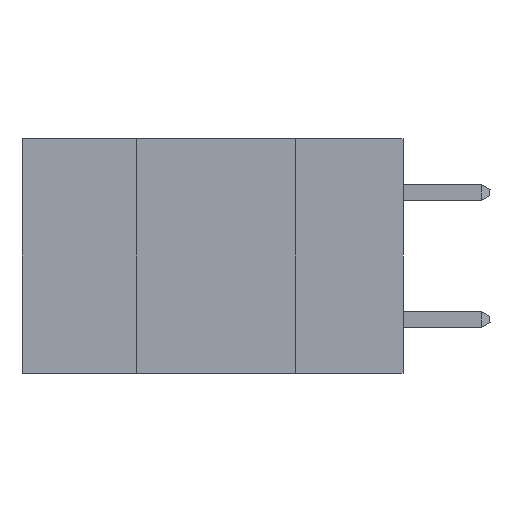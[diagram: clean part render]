
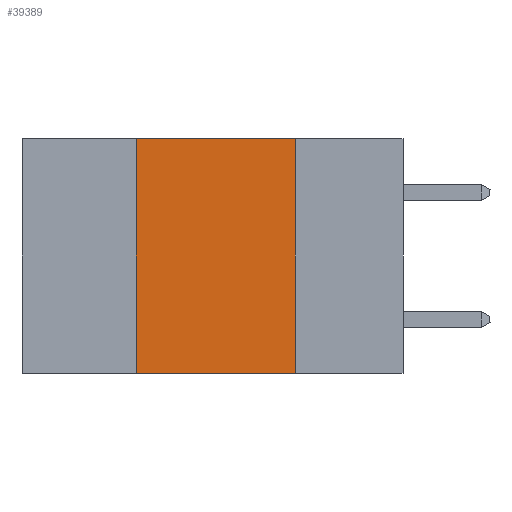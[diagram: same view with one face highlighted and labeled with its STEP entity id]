
A CAD part, left-side view. The second image highlights one B-rep face of the part: STEP entity #39389.
In plain terms, the highlighted planar face has unit normal (-1, 0, 0).
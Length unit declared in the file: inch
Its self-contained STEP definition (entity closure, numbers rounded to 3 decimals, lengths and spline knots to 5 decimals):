
#234 = CARTESIAN_POINT ( 'NONE',  ( 0., 0.6, 0. ) ) ;
#533 = PLANE ( 'NONE',  #46203 ) ;
#936 = ORIENTED_EDGE ( 'NONE', *, *, #8516, .T. ) ;
#1502 = ORIENTED_EDGE ( 'NONE', *, *, #2076, .F. ) ;
#1840 = EDGE_LOOP ( 'NONE', ( #38169, #26956, #1502, #936 ) ) ;
#2076 = EDGE_CURVE ( 'NONE', #39850, #3855, #32888, .T. ) ;
#2745 = DIRECTION ( 'NONE',  ( 0., 0., -1. ) ) ;
#3281 = CARTESIAN_POINT ( 'NONE',  ( 0., 0.17, -0.37 ) ) ;
#3855 = VERTEX_POINT ( 'NONE', #32870 ) ;
#5832 = DIRECTION ( 'NONE',  ( 0., -1., 0. ) ) ;
#7295 = DIRECTION ( 'NONE',  ( 0., -1., 0. ) ) ;
#8516 = EDGE_CURVE ( 'NONE', #39850, #12502, #23339, .T. ) ;
#12502 = VERTEX_POINT ( 'NONE', #3281 ) ;
#12785 = CARTESIAN_POINT ( 'NONE',  ( 0., 0.6, -0.37 ) ) ;
#13663 = VECTOR ( 'NONE', #21708, 39.37008 ) ;
#14873 = VECTOR ( 'NONE', #5832, 39.37008 ) ;
#16962 = CARTESIAN_POINT ( 'NONE',  ( 0., 0.42, -0.37 ) ) ;
#18075 = CARTESIAN_POINT ( 'NONE',  ( 0., 0.42, 0. ) ) ;
#19120 = EDGE_CURVE ( 'NONE', #3855, #32318, #36727, .T. ) ;
#21708 = DIRECTION ( 'NONE',  ( 0., 0., 1. ) ) ;
#23339 = LINE ( 'NONE', #12785, #14873 ) ;
#25687 = DIRECTION ( 'NONE',  ( 0., 0., -1. ) ) ;
#26317 = CARTESIAN_POINT ( 'NONE',  ( 0., 0.17, 0. ) ) ;
#26956 = ORIENTED_EDGE ( 'NONE', *, *, #19120, .F. ) ;
#31053 = VECTOR ( 'NONE', #7295, 39.37008 ) ;
#32318 = VERTEX_POINT ( 'NONE', #26317 ) ;
#32870 = CARTESIAN_POINT ( 'NONE',  ( 0., 0.42, 0. ) ) ;
#32888 = LINE ( 'NONE', #18075, #13663 ) ;
#35145 = CARTESIAN_POINT ( 'NONE',  ( 0., 0.17, 0. ) ) ;
#35933 = CARTESIAN_POINT ( 'NONE',  ( 0., 0.6, 0. ) ) ;
#36727 = LINE ( 'NONE', #35933, #31053 ) ;
#36884 = VECTOR ( 'NONE', #2745, 39.37008 ) ;
#38169 = ORIENTED_EDGE ( 'NONE', *, *, #42313, .F. ) ;
#39389 = ADVANCED_FACE ( 'NONE', ( #40237 ), #533, .F. ) ;
#39850 = VERTEX_POINT ( 'NONE', #16962 ) ;
#40237 = FACE_OUTER_BOUND ( 'NONE', #1840, .T. ) ;
#42313 = EDGE_CURVE ( 'NONE', #32318, #12502, #46452, .T. ) ;
#43314 = DIRECTION ( 'NONE',  ( 1., 0., 0. ) ) ;
#46203 = AXIS2_PLACEMENT_3D ( 'NONE', #234, #43314, #25687 ) ;
#46452 = LINE ( 'NONE', #35145, #36884 ) ;
